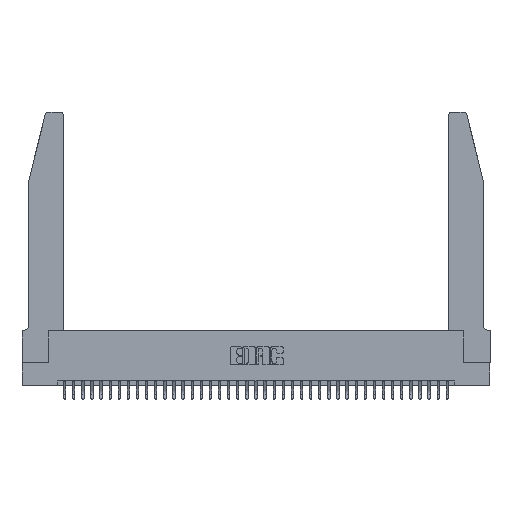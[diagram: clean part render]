
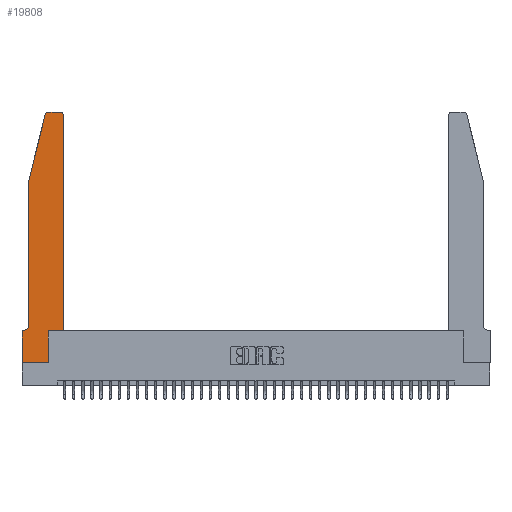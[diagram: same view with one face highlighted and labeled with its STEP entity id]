
A CAD part, top view. The second image highlights one B-rep face of the part: STEP entity #19808.
In plain terms, the highlighted planar face has unit normal (0, 0, 1).
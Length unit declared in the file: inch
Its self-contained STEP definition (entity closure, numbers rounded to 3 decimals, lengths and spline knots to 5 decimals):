
#1356 = ORIENTED_EDGE ( 'NONE', *, *, #28522, .T. ) ;
#1644 = EDGE_CURVE ( 'NONE', #12950, #4197, #7264, .T. ) ;
#1718 = VERTEX_POINT ( 'NONE', #26056 ) ;
#2103 = CARTESIAN_POINT ( 'NONE',  ( 0.4505, 0.35, 0.37 ) ) ;
#2147 = CARTESIAN_POINT ( 'NONE',  ( 0., 0., 0.37 ) ) ;
#2420 = DIRECTION ( 'NONE',  ( 0., -1., 0. ) ) ;
#2650 = EDGE_CURVE ( 'NONE', #15804, #26012, #31459, .T. ) ;
#2767 = LINE ( 'NONE', #9930, #35382 ) ;
#3192 = ORIENTED_EDGE ( 'NONE', *, *, #26631, .T. ) ;
#3567 = ORIENTED_EDGE ( 'NONE', *, *, #1644, .T. ) ;
#3662 = VERTEX_POINT ( 'NONE', #26503 ) ;
#3785 = CIRCLE ( 'NONE', #14761, 0.07 ) ;
#4197 = VERTEX_POINT ( 'NONE', #21029 ) ;
#4486 = AXIS2_PLACEMENT_3D ( 'NONE', #5040, #31849, #25838 ) ;
#5040 = CARTESIAN_POINT ( 'NONE',  ( 0.4205, 2.72, 0.37 ) ) ;
#5110 = EDGE_CURVE ( 'NONE', #26012, #3662, #28128, .T. ) ;
#5126 = DIRECTION ( 'NONE',  ( 0., 1., 0. ) ) ;
#5349 = CARTESIAN_POINT ( 'NONE',  ( 0., 0.35, 0.37 ) ) ;
#6557 = ORIENTED_EDGE ( 'NONE', *, *, #8550, .T. ) ;
#7020 = ORIENTED_EDGE ( 'NONE', *, *, #18956, .T. ) ;
#7264 = LINE ( 'NONE', #29204, #35178 ) ;
#8392 = LINE ( 'NONE', #36839, #21872 ) ;
#8550 = EDGE_CURVE ( 'NONE', #11376, #15241, #38179, .T. ) ;
#8798 = AXIS2_PLACEMENT_3D ( 'NONE', #14278, #29096, #11275 ) ;
#9099 = VECTOR ( 'NONE', #28427, 39.37008 ) ;
#9666 = EDGE_CURVE ( 'NONE', #15241, #15804, #11551, .T. ) ;
#9930 = CARTESIAN_POINT ( 'NONE',  ( 0.2865, 0.35, 0.37 ) ) ;
#10710 = DIRECTION ( 'NONE',  ( 0., 0., -1. ) ) ;
#10780 = CARTESIAN_POINT ( 'NONE',  ( 0.2865, 0., 0.37 ) ) ;
#11078 = CARTESIAN_POINT ( 'NONE',  ( 0.4205, 2.75, 0.37 ) ) ;
#11099 = VECTOR ( 'NONE', #16762, 39.37008 ) ;
#11195 = DIRECTION ( 'NONE',  ( 0., 0., 1. ) ) ;
#11275 = DIRECTION ( 'NONE',  ( 1., 0., 0. ) ) ;
#11376 = VERTEX_POINT ( 'NONE', #11078 ) ;
#11551 = CIRCLE ( 'NONE', #8798, 0.03 ) ;
#11865 = ORIENTED_EDGE ( 'NONE', *, *, #37652, .T. ) ;
#12950 = VERTEX_POINT ( 'NONE', #14242 ) ;
#13702 = ORIENTED_EDGE ( 'NONE', *, *, #5110, .T. ) ;
#13867 = CARTESIAN_POINT ( 'NONE',  ( 0.0755, 2., 0.37 ) ) ;
#14242 = CARTESIAN_POINT ( 'NONE',  ( 0.4505, 0.35, 0.37 ) ) ;
#14278 = CARTESIAN_POINT ( 'NONE',  ( 0.284, 2.72, 0.37 ) ) ;
#14607 = DIRECTION ( 'NONE',  ( 1., 0., 0. ) ) ;
#14761 = AXIS2_PLACEMENT_3D ( 'NONE', #19553, #10710, #19429 ) ;
#14831 = CIRCLE ( 'NONE', #4486, 0.03 ) ;
#15241 = VERTEX_POINT ( 'NONE', #34042 ) ;
#15744 = CARTESIAN_POINT ( 'NONE',  ( 0.0755, 2., 0.37 ) ) ;
#15804 = VERTEX_POINT ( 'NONE', #32653 ) ;
#16762 = DIRECTION ( 'NONE',  ( 1., 0., 0. ) ) ;
#17300 = EDGE_LOOP ( 'NONE', ( #6557, #35642, #20519, #13702, #3192, #1356, #29842, #11865, #25130, #34497, #3567, #7020 ) ) ;
#17863 = EDGE_CURVE ( 'NONE', #37699, #37765, #2767, .T. ) ;
#18358 = VECTOR ( 'NONE', #2420, 39.37008 ) ;
#18548 = DIRECTION ( 'NONE',  ( 0., -1., 0. ) ) ;
#18740 = DIRECTION ( 'NONE',  ( -1., 0., 0. ) ) ;
#18956 = EDGE_CURVE ( 'NONE', #4197, #11376, #14831, .T. ) ;
#19090 = VECTOR ( 'NONE', #22563, 39.37008 ) ;
#19429 = DIRECTION ( 'NONE',  ( -1., 0., 0. ) ) ;
#19436 = VECTOR ( 'NONE', #18548, 39.37008 ) ;
#19553 = CARTESIAN_POINT ( 'NONE',  ( 0.0055, 0.42, 0.37 ) ) ;
#19808 = ADVANCED_FACE ( 'NONE', ( #35732 ), #29426, .T. ) ;
#20519 = ORIENTED_EDGE ( 'NONE', *, *, #2650, .T. ) ;
#21029 = CARTESIAN_POINT ( 'NONE',  ( 0.4505, 2.72, 0.37 ) ) ;
#21488 = AXIS2_PLACEMENT_3D ( 'NONE', #5349, #11195, #14607 ) ;
#21872 = VECTOR ( 'NONE', #18740, 39.37008 ) ;
#22244 = LINE ( 'NONE', #27251, #19436 ) ;
#22563 = DIRECTION ( 'NONE',  ( 1., 0., 0. ) ) ;
#24043 = VERTEX_POINT ( 'NONE', #34380 ) ;
#24972 = DIRECTION ( 'NONE',  ( -1., 0., 0. ) ) ;
#25130 = ORIENTED_EDGE ( 'NONE', *, *, #17863, .T. ) ;
#25838 = DIRECTION ( 'NONE',  ( 1., 0., 0. ) ) ;
#26012 = VERTEX_POINT ( 'NONE', #13867 ) ;
#26056 = CARTESIAN_POINT ( 'NONE',  ( 0., 0., 0.37 ) ) ;
#26503 = CARTESIAN_POINT ( 'NONE',  ( 0.0755, 0.42, 0.37 ) ) ;
#26631 = EDGE_CURVE ( 'NONE', #3662, #24043, #3785, .T. ) ;
#27161 = CARTESIAN_POINT ( 'NONE',  ( 0.2605, 2.75, 0.37 ) ) ;
#27251 = CARTESIAN_POINT ( 'NONE',  ( 0., 0., 0.37 ) ) ;
#27655 = VERTEX_POINT ( 'NONE', #36292 ) ;
#28128 = LINE ( 'NONE', #15744, #18358 ) ;
#28427 = DIRECTION ( 'NONE',  ( -0.239, -0.971, 0. ) ) ;
#28522 = EDGE_CURVE ( 'NONE', #24043, #27655, #8392, .T. ) ;
#29044 = CARTESIAN_POINT ( 'NONE',  ( 0.2865, 0.35, 0.37 ) ) ;
#29096 = DIRECTION ( 'NONE',  ( 0., 0., 1. ) ) ;
#29204 = CARTESIAN_POINT ( 'NONE',  ( 0.4505, 0.35, 0.37 ) ) ;
#29322 = VECTOR ( 'NONE', #24972, 39.37008 ) ;
#29426 = PLANE ( 'NONE',  #21488 ) ;
#29821 = LINE ( 'NONE', #2103, #19090 ) ;
#29842 = ORIENTED_EDGE ( 'NONE', *, *, #33302, .T. ) ;
#30831 = CARTESIAN_POINT ( 'NONE',  ( 0.0755, 2., 0.37 ) ) ;
#31459 = LINE ( 'NONE', #30831, #9099 ) ;
#31849 = DIRECTION ( 'NONE',  ( 0., 0., 1. ) ) ;
#32653 = CARTESIAN_POINT ( 'NONE',  ( 0.25487, 2.72718, 0.37 ) ) ;
#33302 = EDGE_CURVE ( 'NONE', #27655, #1718, #22244, .T. ) ;
#34042 = CARTESIAN_POINT ( 'NONE',  ( 0.284, 2.75, 0.37 ) ) ;
#34261 = DIRECTION ( 'NONE',  ( 0., 1., 0. ) ) ;
#34380 = CARTESIAN_POINT ( 'NONE',  ( 0.0055, 0.35, 0.37 ) ) ;
#34497 = ORIENTED_EDGE ( 'NONE', *, *, #36457, .T. ) ;
#35178 = VECTOR ( 'NONE', #5126, 39.37008 ) ;
#35382 = VECTOR ( 'NONE', #34261, 39.37008 ) ;
#35642 = ORIENTED_EDGE ( 'NONE', *, *, #9666, .T. ) ;
#35732 = FACE_OUTER_BOUND ( 'NONE', #17300, .T. ) ;
#36292 = CARTESIAN_POINT ( 'NONE',  ( 0., 0.35, 0.37 ) ) ;
#36457 = EDGE_CURVE ( 'NONE', #37765, #12950, #29821, .T. ) ;
#36839 = CARTESIAN_POINT ( 'NONE',  ( 0.0755, 0.35, 0.37 ) ) ;
#37652 = EDGE_CURVE ( 'NONE', #1718, #37699, #38106, .T. ) ;
#37699 = VERTEX_POINT ( 'NONE', #10780 ) ;
#37765 = VERTEX_POINT ( 'NONE', #29044 ) ;
#38106 = LINE ( 'NONE', #2147, #11099 ) ;
#38179 = LINE ( 'NONE', #27161, #29322 ) ;
